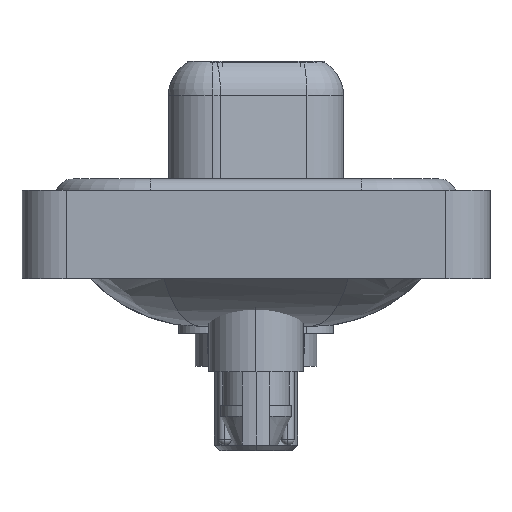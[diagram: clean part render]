
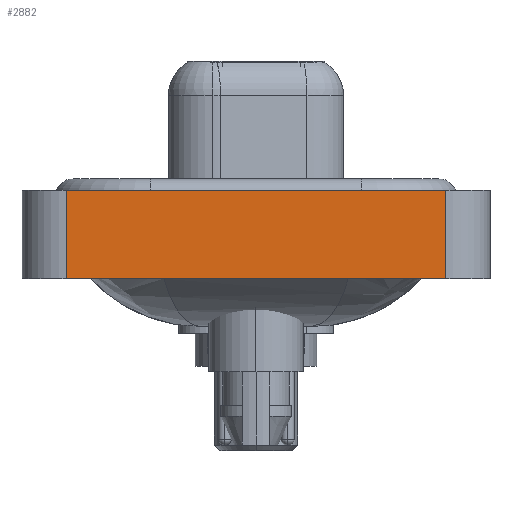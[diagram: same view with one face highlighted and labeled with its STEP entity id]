
A CAD part, left-side view. The second image highlights one B-rep face of the part: STEP entity #2882.
In plain terms, the highlighted planar face has unit normal (-1, 0, 0).
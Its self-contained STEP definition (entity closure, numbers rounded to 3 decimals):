
#437 = DIRECTION ( 'NONE',  ( 0., -1., 0. ) ) ;
#663 = CARTESIAN_POINT ( 'NONE',  ( -7.35, -8.55, -3.6 ) ) ;
#672 = VERTEX_POINT ( 'NONE', #14348 ) ;
#2810 = AXIS2_PLACEMENT_3D ( 'NONE', #18801, #27768, #23569 ) ;
#2882 = ADVANCED_FACE ( 'NONE', ( #18942 ), #14841, .T. ) ;
#3121 = VERTEX_POINT ( 'NONE', #9602 ) ;
#3623 = EDGE_CURVE ( 'NONE', #3121, #672, #13638, .T. ) ;
#3772 = EDGE_LOOP ( 'NONE', ( #25921, #7019, #22193, #20552 ) ) ;
#3991 = EDGE_CURVE ( 'NONE', #25520, #3121, #9110, .T. ) ;
#5823 = CARTESIAN_POINT ( 'NONE',  ( -7.35, 8.55, -3.6 ) ) ;
#6014 = CARTESIAN_POINT ( 'NONE',  ( -7.35, 8.55, -3.6 ) ) ;
#6657 = CARTESIAN_POINT ( 'NONE',  ( -7.35, 8.55, 0.4 ) ) ;
#7019 = ORIENTED_EDGE ( 'NONE', *, *, #23822, .F. ) ;
#9110 = LINE ( 'NONE', #663, #25914 ) ;
#9258 = DIRECTION ( 'NONE',  ( 0., -1., 0. ) ) ;
#9424 = DIRECTION ( 'NONE',  ( 0., 0., 1. ) ) ;
#9602 = CARTESIAN_POINT ( 'NONE',  ( -7.35, -8.55, -3.6 ) ) ;
#9790 = LINE ( 'NONE', #5823, #17757 ) ;
#10389 = EDGE_CURVE ( 'NONE', #25520, #26642, #9790, .T. ) ;
#11783 = VECTOR ( 'NONE', #437, 1000. ) ;
#13638 = LINE ( 'NONE', #24040, #23669 ) ;
#14348 = CARTESIAN_POINT ( 'NONE',  ( -7.35, -8.55, 0.4 ) ) ;
#14841 = PLANE ( 'NONE',  #2810 ) ;
#17757 = VECTOR ( 'NONE', #20745, 1000. ) ;
#18801 = CARTESIAN_POINT ( 'NONE',  ( -7.35, -8.55, -3.6 ) ) ;
#18942 = FACE_OUTER_BOUND ( 'NONE', #3772, .T. ) ;
#19724 = LINE ( 'NONE', #19853, #11783 ) ;
#19853 = CARTESIAN_POINT ( 'NONE',  ( -7.35, -8.55, 0.4 ) ) ;
#20552 = ORIENTED_EDGE ( 'NONE', *, *, #3991, .T. ) ;
#20745 = DIRECTION ( 'NONE',  ( 0., 0., 1. ) ) ;
#22193 = ORIENTED_EDGE ( 'NONE', *, *, #10389, .F. ) ;
#23569 = DIRECTION ( 'NONE',  ( 0., 0., 1. ) ) ;
#23669 = VECTOR ( 'NONE', #9424, 1000. ) ;
#23822 = EDGE_CURVE ( 'NONE', #26642, #672, #19724, .T. ) ;
#24040 = CARTESIAN_POINT ( 'NONE',  ( -7.35, -8.55, -3.6 ) ) ;
#25520 = VERTEX_POINT ( 'NONE', #6014 ) ;
#25914 = VECTOR ( 'NONE', #9258, 1000. ) ;
#25921 = ORIENTED_EDGE ( 'NONE', *, *, #3623, .T. ) ;
#26642 = VERTEX_POINT ( 'NONE', #6657 ) ;
#27768 = DIRECTION ( 'NONE',  ( -1., 0., 0. ) ) ;
